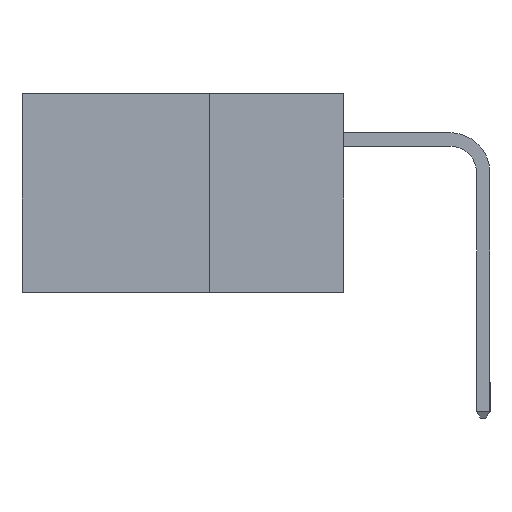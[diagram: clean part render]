
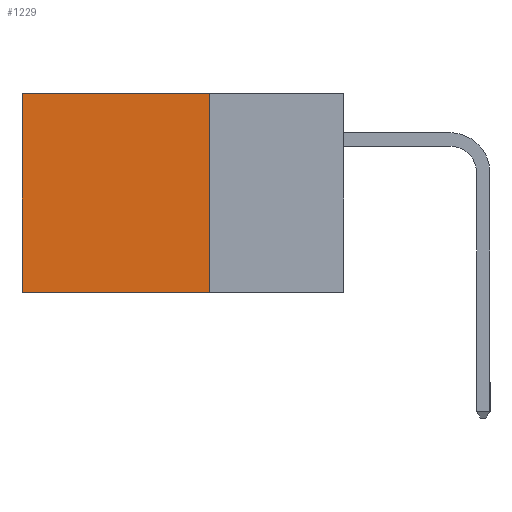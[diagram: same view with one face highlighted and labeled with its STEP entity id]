
A CAD part, left-side view. The second image highlights one B-rep face of the part: STEP entity #1229.
In plain terms, the highlighted planar face has unit normal (-1, 0, 0).
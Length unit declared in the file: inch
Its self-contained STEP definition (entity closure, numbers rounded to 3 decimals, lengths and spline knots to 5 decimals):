
#276 = VECTOR ( 'NONE', #8974, 39.37008 ) ;
#862 = EDGE_CURVE ( 'NONE', #7573, #11878, #8268, .T. ) ;
#1229 = ADVANCED_FACE ( 'NONE', ( #17290 ), #3201, .F. ) ;
#1603 = VECTOR ( 'NONE', #4222, 39.37008 ) ;
#2111 = EDGE_CURVE ( 'NONE', #10022, #10977, #9413, .T. ) ;
#3201 = PLANE ( 'NONE',  #8247 ) ;
#3206 = ORIENTED_EDGE ( 'NONE', *, *, #862, .T. ) ;
#3892 = CARTESIAN_POINT ( 'NONE',  ( 0.298, 0.25, 0. ) ) ;
#4062 = CARTESIAN_POINT ( 'NONE',  ( 0.298, 0.6, 0. ) ) ;
#4087 = CARTESIAN_POINT ( 'NONE',  ( 0.298, 0.25, 0. ) ) ;
#4222 = DIRECTION ( 'NONE',  ( 0., 1., 0. ) ) ;
#4983 = EDGE_CURVE ( 'NONE', #10022, #7573, #9592, .T. ) ;
#6226 = ORIENTED_EDGE ( 'NONE', *, *, #4983, .T. ) ;
#6848 = CARTESIAN_POINT ( 'NONE',  ( 0.298, 0.25, -0.37 ) ) ;
#7573 = VERTEX_POINT ( 'NONE', #10992 ) ;
#7814 = ORIENTED_EDGE ( 'NONE', *, *, #17775, .F. ) ;
#8247 = AXIS2_PLACEMENT_3D ( 'NONE', #17547, #18985, #16976 ) ;
#8268 = LINE ( 'NONE', #4062, #276 ) ;
#8974 = DIRECTION ( 'NONE',  ( 0., 0., -1. ) ) ;
#9224 = EDGE_LOOP ( 'NONE', ( #3206, #7814, #14637, #6226 ) ) ;
#9413 = LINE ( 'NONE', #4087, #13744 ) ;
#9461 = VECTOR ( 'NONE', #15655, 39.37008 ) ;
#9592 = LINE ( 'NONE', #17987, #1603 ) ;
#10022 = VERTEX_POINT ( 'NONE', #3892 ) ;
#10385 = LINE ( 'NONE', #6848, #9461 ) ;
#10977 = VERTEX_POINT ( 'NONE', #19031 ) ;
#10992 = CARTESIAN_POINT ( 'NONE',  ( 0.298, 0.6, 0. ) ) ;
#11064 = CARTESIAN_POINT ( 'NONE',  ( 0.298, 0.6, -0.37 ) ) ;
#11878 = VERTEX_POINT ( 'NONE', #11064 ) ;
#13744 = VECTOR ( 'NONE', #16230, 39.37008 ) ;
#14637 = ORIENTED_EDGE ( 'NONE', *, *, #2111, .F. ) ;
#15655 = DIRECTION ( 'NONE',  ( 0., 1., 0. ) ) ;
#16230 = DIRECTION ( 'NONE',  ( 0., 0., -1. ) ) ;
#16976 = DIRECTION ( 'NONE',  ( 0., 0., -1. ) ) ;
#17290 = FACE_OUTER_BOUND ( 'NONE', #9224, .T. ) ;
#17547 = CARTESIAN_POINT ( 'NONE',  ( 0.298, 0.25, 0. ) ) ;
#17775 = EDGE_CURVE ( 'NONE', #10977, #11878, #10385, .T. ) ;
#17987 = CARTESIAN_POINT ( 'NONE',  ( 0.298, 0.25, 0. ) ) ;
#18985 = DIRECTION ( 'NONE',  ( 1., 0., 0. ) ) ;
#19031 = CARTESIAN_POINT ( 'NONE',  ( 0.298, 0.25, -0.37 ) ) ;
